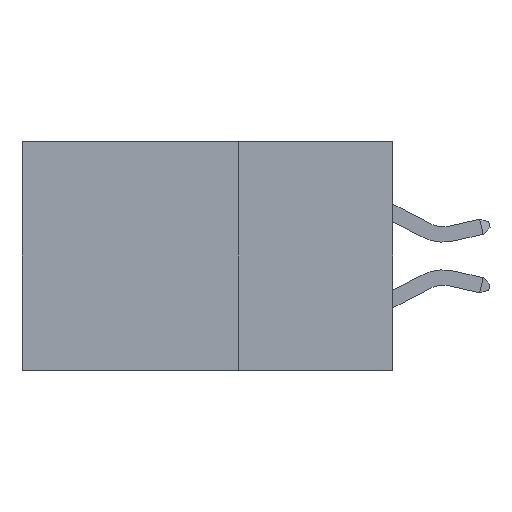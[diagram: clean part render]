
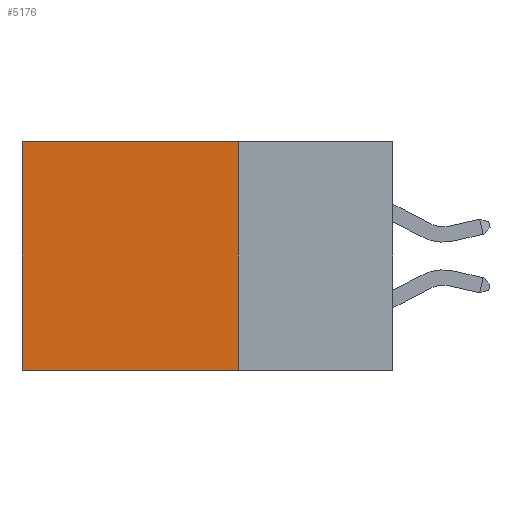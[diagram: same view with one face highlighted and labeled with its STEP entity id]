
A CAD part, left-side view. The second image highlights one B-rep face of the part: STEP entity #5176.
In plain terms, the highlighted planar face has unit normal (-1, 0, 0).
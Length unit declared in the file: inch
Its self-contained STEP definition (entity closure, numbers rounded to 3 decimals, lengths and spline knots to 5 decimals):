
#301 = EDGE_CURVE ( 'NONE', #8681, #10675, #14403, .T. ) ;
#1157 = VECTOR ( 'NONE', #1933, 39.37008 ) ;
#1363 = PLANE ( 'NONE',  #6892 ) ;
#1933 = DIRECTION ( 'NONE',  ( 0., 0., -1. ) ) ;
#2207 = LINE ( 'NONE', #6604, #10632 ) ;
#3016 = CARTESIAN_POINT ( 'NONE',  ( 0.2875, 0.25, 0. ) ) ;
#3617 = DIRECTION ( 'NONE',  ( 0., 0., -1. ) ) ;
#5004 = CARTESIAN_POINT ( 'NONE',  ( 0.2875, 0.6, 0. ) ) ;
#5176 = ADVANCED_FACE ( 'NONE', ( #11583 ), #1363, .F. ) ;
#5619 = VECTOR ( 'NONE', #7260, 39.37008 ) ;
#5851 = ORIENTED_EDGE ( 'NONE', *, *, #8145, .T. ) ;
#6604 = CARTESIAN_POINT ( 'NONE',  ( 0.2875, 0.25, -0.37 ) ) ;
#6892 = AXIS2_PLACEMENT_3D ( 'NONE', #10528, #13902, #9194 ) ;
#7260 = DIRECTION ( 'NONE',  ( 0., 1., 0. ) ) ;
#8145 = EDGE_CURVE ( 'NONE', #10002, #8681, #12109, .T. ) ;
#8579 = CARTESIAN_POINT ( 'NONE',  ( 0.2875, 0.6, 0. ) ) ;
#8680 = CARTESIAN_POINT ( 'NONE',  ( 0.2875, 0.6, -0.37 ) ) ;
#8681 = VERTEX_POINT ( 'NONE', #5004 ) ;
#9154 = EDGE_CURVE ( 'NONE', #11128, #10675, #2207, .T. ) ;
#9194 = DIRECTION ( 'NONE',  ( 0., 0., -1. ) ) ;
#9447 = VECTOR ( 'NONE', #3617, 39.37008 ) ;
#10002 = VERTEX_POINT ( 'NONE', #3016 ) ;
#10383 = EDGE_LOOP ( 'NONE', ( #10561, #11553, #11954, #5851 ) ) ;
#10406 = LINE ( 'NONE', #13851, #9447 ) ;
#10528 = CARTESIAN_POINT ( 'NONE',  ( 0.2875, 0.25, 0. ) ) ;
#10561 = ORIENTED_EDGE ( 'NONE', *, *, #301, .T. ) ;
#10632 = VECTOR ( 'NONE', #11096, 39.37008 ) ;
#10675 = VERTEX_POINT ( 'NONE', #8680 ) ;
#11096 = DIRECTION ( 'NONE',  ( 0., 1., 0. ) ) ;
#11128 = VERTEX_POINT ( 'NONE', #11737 ) ;
#11553 = ORIENTED_EDGE ( 'NONE', *, *, #9154, .F. ) ;
#11583 = FACE_OUTER_BOUND ( 'NONE', #10383, .T. ) ;
#11737 = CARTESIAN_POINT ( 'NONE',  ( 0.2875, 0.25, -0.37 ) ) ;
#11954 = ORIENTED_EDGE ( 'NONE', *, *, #12213, .F. ) ;
#12109 = LINE ( 'NONE', #12179, #5619 ) ;
#12179 = CARTESIAN_POINT ( 'NONE',  ( 0.2875, 0.25, 0. ) ) ;
#12213 = EDGE_CURVE ( 'NONE', #10002, #11128, #10406, .T. ) ;
#13851 = CARTESIAN_POINT ( 'NONE',  ( 0.2875, 0.25, 0. ) ) ;
#13902 = DIRECTION ( 'NONE',  ( 1., 0., 0. ) ) ;
#14403 = LINE ( 'NONE', #8579, #1157 ) ;
